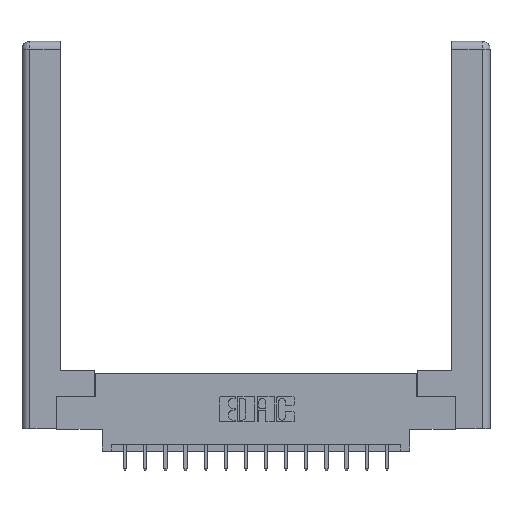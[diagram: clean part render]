
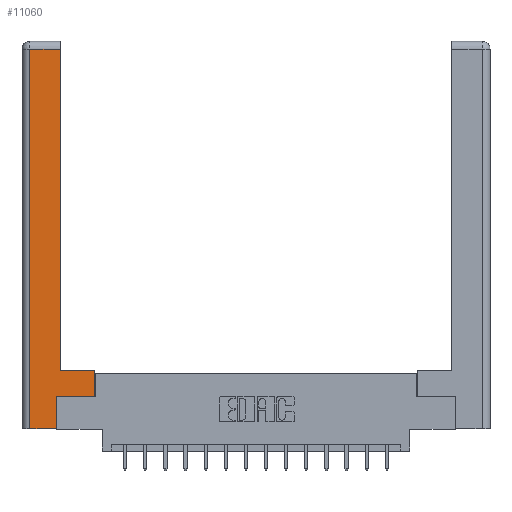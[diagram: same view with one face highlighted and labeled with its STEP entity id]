
A CAD part, top view. The second image highlights one B-rep face of the part: STEP entity #11060.
In plain terms, the highlighted planar face has unit normal (0, 0, 1).
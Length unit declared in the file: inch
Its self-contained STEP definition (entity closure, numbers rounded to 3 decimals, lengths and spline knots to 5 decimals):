
#48 = EDGE_CURVE ( 'NONE', #9711, #14444, #4654, .T. ) ;
#258 = AXIS2_PLACEMENT_3D ( 'NONE', #9564, #10817, #17051 ) ;
#289 = DIRECTION ( 'NONE',  ( -1., 0., 0. ) ) ;
#331 = CARTESIAN_POINT ( 'NONE',  ( 0.295, 2.94, 0. ) ) ;
#413 = VECTOR ( 'NONE', #11071, 39.37008 ) ;
#535 = VECTOR ( 'NONE', #3526, 39.37008 ) ;
#760 = VECTOR ( 'NONE', #289, 39.37008 ) ;
#995 = EDGE_CURVE ( 'NONE', #10910, #3928, #3461, .T. ) ;
#1059 = VERTEX_POINT ( 'NONE', #331 ) ;
#1501 = CARTESIAN_POINT ( 'NONE',  ( 0.565, 0.45, 0. ) ) ;
#1513 = CARTESIAN_POINT ( 'NONE',  ( 0.565, 0.245, 0. ) ) ;
#1807 = EDGE_CURVE ( 'NONE', #2101, #1935, #14569, .T. ) ;
#1831 = DIRECTION ( 'NONE',  ( 0., 1., 0. ) ) ;
#1935 = VERTEX_POINT ( 'NONE', #12939 ) ;
#2101 = VERTEX_POINT ( 'NONE', #1501 ) ;
#2875 = LINE ( 'NONE', #7167, #16673 ) ;
#3057 = DIRECTION ( 'NONE',  ( 0., 1., 0. ) ) ;
#3461 = LINE ( 'NONE', #5619, #9808 ) ;
#3526 = DIRECTION ( 'NONE',  ( 0., -1., 0. ) ) ;
#3724 = CARTESIAN_POINT ( 'NONE',  ( 0.0615, 0., 0. ) ) ;
#3928 = VERTEX_POINT ( 'NONE', #4850 ) ;
#4093 = VECTOR ( 'NONE', #3057, 39.37008 ) ;
#4121 = CARTESIAN_POINT ( 'NONE',  ( 0.295, 0.45, 0. ) ) ;
#4257 = CARTESIAN_POINT ( 'NONE',  ( 0.295, 3., 0. ) ) ;
#4479 = LINE ( 'NONE', #12861, #12720 ) ;
#4654 = LINE ( 'NONE', #9705, #413 ) ;
#4715 = LINE ( 'NONE', #12652, #4093 ) ;
#4850 = CARTESIAN_POINT ( 'NONE',  ( 0.265, 0., 0. ) ) ;
#5619 = CARTESIAN_POINT ( 'NONE',  ( 0.265, 0., 0. ) ) ;
#5772 = FACE_OUTER_BOUND ( 'NONE', #5845, .T. ) ;
#5845 = EDGE_LOOP ( 'NONE', ( #8181, #11395, #9869, #16169, #14299, #9174, #9339, #10651 ) ) ;
#7167 = CARTESIAN_POINT ( 'NONE',  ( 0.265, 0.245, 0. ) ) ;
#8135 = EDGE_CURVE ( 'NONE', #1935, #1059, #11750, .T. ) ;
#8181 = ORIENTED_EDGE ( 'NONE', *, *, #8135, .T. ) ;
#8190 = VECTOR ( 'NONE', #13650, 39.37008 ) ;
#9174 = ORIENTED_EDGE ( 'NONE', *, *, #48, .T. ) ;
#9339 = ORIENTED_EDGE ( 'NONE', *, *, #10021, .T. ) ;
#9564 = CARTESIAN_POINT ( 'NONE',  ( 0., 0., 0. ) ) ;
#9705 = CARTESIAN_POINT ( 'NONE',  ( 0.565, 0.245, 0. ) ) ;
#9711 = VERTEX_POINT ( 'NONE', #14584 ) ;
#9799 = VERTEX_POINT ( 'NONE', #16009 ) ;
#9808 = VECTOR ( 'NONE', #13719, 39.37008 ) ;
#9869 = ORIENTED_EDGE ( 'NONE', *, *, #14725, .T. ) ;
#10021 = EDGE_CURVE ( 'NONE', #14444, #2101, #4715, .T. ) ;
#10440 = CARTESIAN_POINT ( 'NONE',  ( 0.0615, 0., 0. ) ) ;
#10651 = ORIENTED_EDGE ( 'NONE', *, *, #1807, .T. ) ;
#10703 = EDGE_CURVE ( 'NONE', #1059, #9799, #4479, .T. ) ;
#10817 = DIRECTION ( 'NONE',  ( 0., 0., -1. ) ) ;
#10910 = VERTEX_POINT ( 'NONE', #3724 ) ;
#11060 = ADVANCED_FACE ( 'NONE', ( #5772 ), #14759, .F. ) ;
#11071 = DIRECTION ( 'NONE',  ( 1., 0., 0. ) ) ;
#11395 = ORIENTED_EDGE ( 'NONE', *, *, #10703, .T. ) ;
#11750 = LINE ( 'NONE', #4257, #8190 ) ;
#12652 = CARTESIAN_POINT ( 'NONE',  ( 0.565, 0.45, 0. ) ) ;
#12720 = VECTOR ( 'NONE', #14063, 39.37008 ) ;
#12734 = EDGE_CURVE ( 'NONE', #3928, #9711, #2875, .T. ) ;
#12861 = CARTESIAN_POINT ( 'NONE',  ( 0.0615, 2.94, 0. ) ) ;
#12939 = CARTESIAN_POINT ( 'NONE',  ( 0.295, 0.45, 0. ) ) ;
#13650 = DIRECTION ( 'NONE',  ( 0., 1., 0. ) ) ;
#13719 = DIRECTION ( 'NONE',  ( 1., 0., 0. ) ) ;
#13726 = LINE ( 'NONE', #10440, #535 ) ;
#14063 = DIRECTION ( 'NONE',  ( -1., 0., 0. ) ) ;
#14299 = ORIENTED_EDGE ( 'NONE', *, *, #12734, .T. ) ;
#14444 = VERTEX_POINT ( 'NONE', #1513 ) ;
#14569 = LINE ( 'NONE', #4121, #760 ) ;
#14584 = CARTESIAN_POINT ( 'NONE',  ( 0.265, 0.245, 0. ) ) ;
#14725 = EDGE_CURVE ( 'NONE', #9799, #10910, #13726, .T. ) ;
#14759 = PLANE ( 'NONE',  #258 ) ;
#16009 = CARTESIAN_POINT ( 'NONE',  ( 0.0615, 2.94, 0. ) ) ;
#16169 = ORIENTED_EDGE ( 'NONE', *, *, #995, .T. ) ;
#16673 = VECTOR ( 'NONE', #1831, 39.37008 ) ;
#17051 = DIRECTION ( 'NONE',  ( -1., 0., 0. ) ) ;
